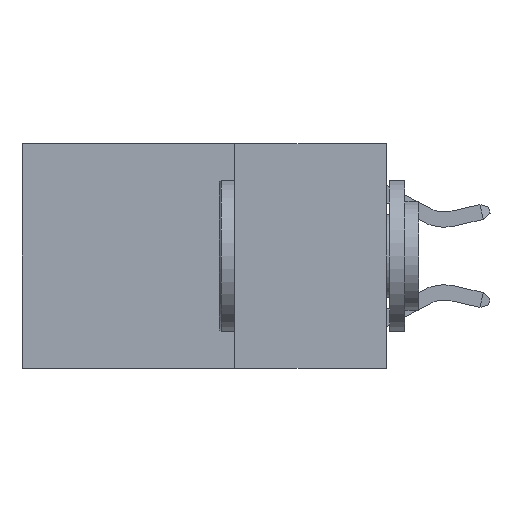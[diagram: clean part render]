
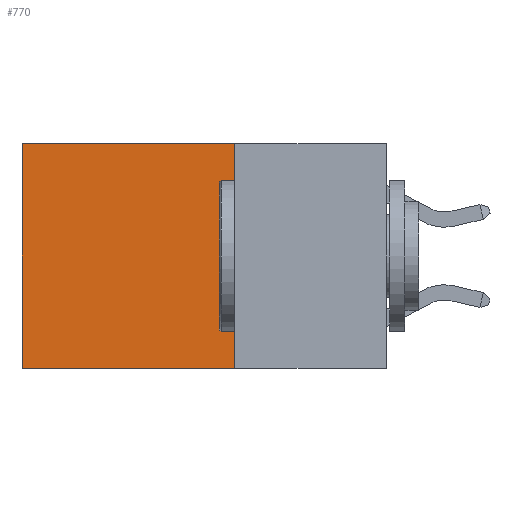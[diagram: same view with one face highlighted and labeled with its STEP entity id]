
A CAD part, left-side view. The second image highlights one B-rep face of the part: STEP entity #770.
In plain terms, the highlighted planar face has unit normal (-1, 0, 0).
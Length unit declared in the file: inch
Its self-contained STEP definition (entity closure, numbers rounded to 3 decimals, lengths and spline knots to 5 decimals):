
#26 = LINE ( 'NONE', #14835, #5395 ) ;
#90 = VECTOR ( 'NONE', #7196, 39.37008 ) ;
#449 = ORIENTED_EDGE ( 'NONE', *, *, #14043, .T. ) ;
#770 = ADVANCED_FACE ( 'NONE', ( #1411 ), #8363, .F. ) ;
#1016 = CARTESIAN_POINT ( 'NONE',  ( 0.2625, 0.6, -0.37 ) ) ;
#1411 = FACE_OUTER_BOUND ( 'NONE', #5114, .T. ) ;
#1603 = LINE ( 'NONE', #7275, #13145 ) ;
#1702 = CARTESIAN_POINT ( 'NONE',  ( 0.2625, 0.6, 0. ) ) ;
#2275 = LINE ( 'NONE', #1702, #5052 ) ;
#2738 = DIRECTION ( 'NONE',  ( 0., 1., 0. ) ) ;
#2848 = CARTESIAN_POINT ( 'NONE',  ( 0.2625, 0.25, 0. ) ) ;
#3473 = LINE ( 'NONE', #6076, #90 ) ;
#3856 = CARTESIAN_POINT ( 'NONE',  ( 0.2625, 0.25, -0.37 ) ) ;
#4619 = CARTESIAN_POINT ( 'NONE',  ( 0.2625, 0.6, 0. ) ) ;
#4801 = VERTEX_POINT ( 'NONE', #2848 ) ;
#5052 = VECTOR ( 'NONE', #7557, 39.37008 ) ;
#5114 = EDGE_LOOP ( 'NONE', ( #11612, #6780, #11102, #449 ) ) ;
#5395 = VECTOR ( 'NONE', #13673, 39.37008 ) ;
#6027 = DIRECTION ( 'NONE',  ( 1., 0., 0. ) ) ;
#6076 = CARTESIAN_POINT ( 'NONE',  ( 0.2625, 0.25, 0. ) ) ;
#6190 = AXIS2_PLACEMENT_3D ( 'NONE', #11926, #6027, #10804 ) ;
#6472 = VERTEX_POINT ( 'NONE', #3856 ) ;
#6780 = ORIENTED_EDGE ( 'NONE', *, *, #12034, .F. ) ;
#7196 = DIRECTION ( 'NONE',  ( 0., 1., 0. ) ) ;
#7275 = CARTESIAN_POINT ( 'NONE',  ( 0.2625, 0.25, -0.37 ) ) ;
#7347 = VERTEX_POINT ( 'NONE', #1016 ) ;
#7557 = DIRECTION ( 'NONE',  ( 0., 0., -1. ) ) ;
#7786 = EDGE_CURVE ( 'NONE', #11787, #7347, #2275, .T. ) ;
#8363 = PLANE ( 'NONE',  #6190 ) ;
#10804 = DIRECTION ( 'NONE',  ( 0., 0., -1. ) ) ;
#11102 = ORIENTED_EDGE ( 'NONE', *, *, #11653, .F. ) ;
#11612 = ORIENTED_EDGE ( 'NONE', *, *, #7786, .T. ) ;
#11653 = EDGE_CURVE ( 'NONE', #4801, #6472, #26, .T. ) ;
#11787 = VERTEX_POINT ( 'NONE', #4619 ) ;
#11926 = CARTESIAN_POINT ( 'NONE',  ( 0.2625, 0.25, 0. ) ) ;
#12034 = EDGE_CURVE ( 'NONE', #6472, #7347, #1603, .T. ) ;
#13145 = VECTOR ( 'NONE', #2738, 39.37008 ) ;
#13673 = DIRECTION ( 'NONE',  ( 0., 0., -1. ) ) ;
#14043 = EDGE_CURVE ( 'NONE', #4801, #11787, #3473, .T. ) ;
#14835 = CARTESIAN_POINT ( 'NONE',  ( 0.2625, 0.25, 0. ) ) ;
